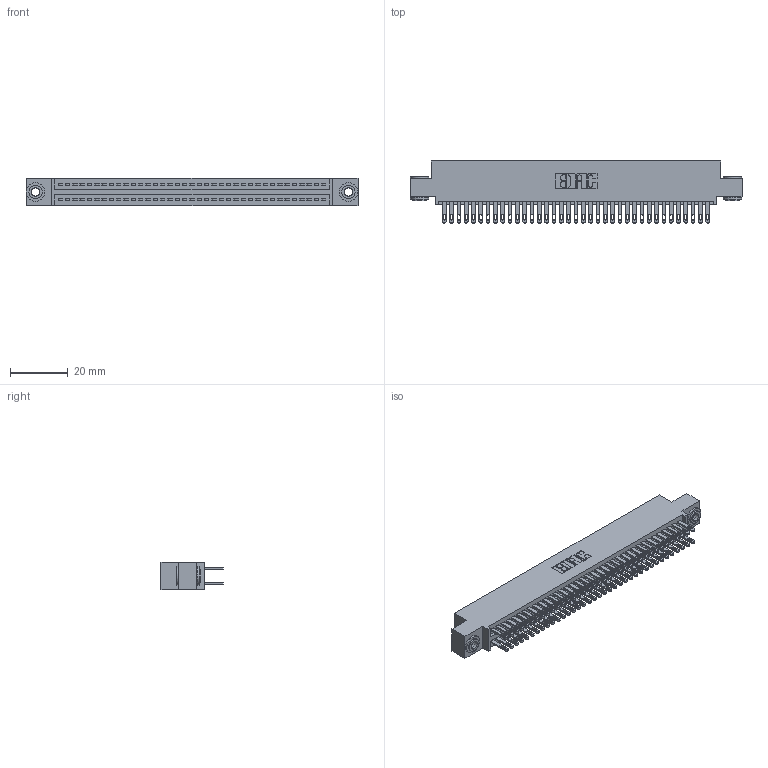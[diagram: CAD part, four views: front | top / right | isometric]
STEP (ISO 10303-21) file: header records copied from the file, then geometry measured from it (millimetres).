
FILE_DESCRIPTION (( 'STEP AP203' ), '1' );
FILE_NAME ('345-074-500-503.STEP', '2018-10-02T10:51:10', ( '' ), ( '' ), 'SwSTEP 2.0', 'SolidWorks 2016', '' );
FILE_SCHEMA (( 'CONFIG_CONTROL_DESIGN' ));
Length unit declared in the file: inch
Products named in the file (4): 345-250-002_345-250-002-102; 345 Part_0.110 Offset - 0.156 Dia-TH; 345-292-001_345-293-100; 345-074-500-503
Assembly tree (77 placements, depth 2):
  345-074-500-503
    345 Part_0.110 Offset - 0.156 Dia-TH
    345-292-001_345-293-100  x74
    345-250-002_345-250-002-102  x2
Bounding box: 115.19 x 21.51 x 9.4 mm (x, y, z)
Volume: 11315.3 mm3; surface area: 17681.6 mm2
Topology: 77 solids, 77 shells, 3572 faces, 10863 edges, 7238 vertices
Faces by surface type: plane 2092, cylinder 1472, cone 8
Entity records: 30416 total; most frequent: CARTESIAN_POINT 5079, ORIENTED_EDGE 5006, DIRECTION 4517, EDGE_CURVE 2503, LINE 2195, VECTOR 2195, VERTEX_POINT 1666, AXIS2_PLACEMENT_3D 1161
